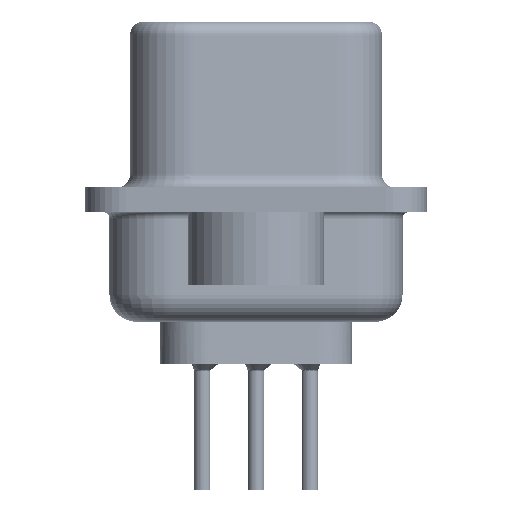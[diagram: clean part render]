
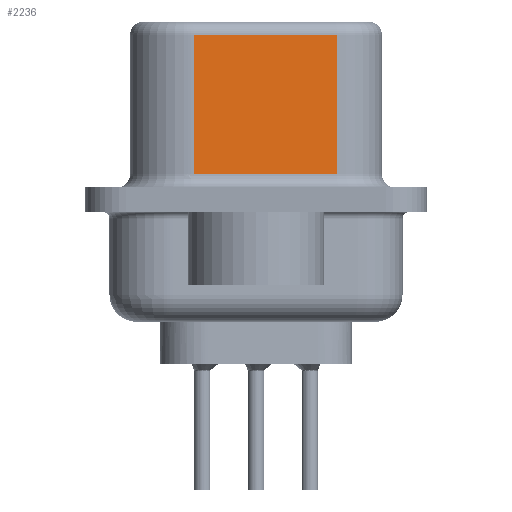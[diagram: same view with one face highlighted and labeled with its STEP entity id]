
A CAD part, left-side view. The second image highlights one B-rep face of the part: STEP entity #2236.
In plain terms, the highlighted planar face has unit normal (-0.985, -0.174, 0).
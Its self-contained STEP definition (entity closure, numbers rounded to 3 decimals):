
#2236 = ADVANCED_FACE ( 'NONE', ( #20825 ), #32775, .F. ) ;
#2850 = LINE ( 'NONE', #18222, #16570 ) ;
#3858 = ORIENTED_EDGE ( 'NONE', *, *, #23259, .T. ) ;
#4111 = EDGE_CURVE ( 'NONE', #20514, #13007, #37584, .T. ) ;
#10504 = CARTESIAN_POINT ( 'NONE',  ( 3.62, 2.293, 0.95 ) ) ;
#12948 = DIRECTION ( 'NONE',  ( 0., 0., -1. ) ) ;
#13007 = VERTEX_POINT ( 'NONE', #10504 ) ;
#13363 = CARTESIAN_POINT ( 'NONE',  ( 4.551, -2.987, 6.07 ) ) ;
#13517 = DIRECTION ( 'NONE',  ( 0., 0., -1. ) ) ;
#13564 = LINE ( 'NONE', #13363, #33303 ) ;
#15489 = VERTEX_POINT ( 'NONE', #37236 ) ;
#16129 = EDGE_CURVE ( 'NONE', #20421, #15489, #35183, .T. ) ;
#16496 = CARTESIAN_POINT ( 'NONE',  ( 4.551, -2.987, 6.57 ) ) ;
#16570 = VECTOR ( 'NONE', #27394, 1000. ) ;
#16953 = EDGE_LOOP ( 'NONE', ( #39284, #33028, #21821, #3858 ) ) ;
#18222 = CARTESIAN_POINT ( 'NONE',  ( 4.551, -2.987, 0.95 ) ) ;
#18298 = CARTESIAN_POINT ( 'NONE',  ( 4.551, -2.987, 6.07 ) ) ;
#20033 = EDGE_CURVE ( 'NONE', #20421, #20514, #13564, .T. ) ;
#20203 = CARTESIAN_POINT ( 'NONE',  ( 3.62, 2.293, 6.07 ) ) ;
#20421 = VERTEX_POINT ( 'NONE', #18298 ) ;
#20514 = VERTEX_POINT ( 'NONE', #20203 ) ;
#20825 = FACE_OUTER_BOUND ( 'NONE', #16953, .T. ) ;
#21821 = ORIENTED_EDGE ( 'NONE', *, *, #4111, .T. ) ;
#23259 = EDGE_CURVE ( 'NONE', #13007, #15489, #2850, .T. ) ;
#24296 = VECTOR ( 'NONE', #12948, 1000. ) ;
#24894 = CARTESIAN_POINT ( 'NONE',  ( 3.62, 2.293, 6.57 ) ) ;
#27004 = DIRECTION ( 'NONE',  ( -0.174, 0.985, 0. ) ) ;
#27394 = DIRECTION ( 'NONE',  ( 0.174, -0.985, 0. ) ) ;
#29694 = VECTOR ( 'NONE', #13517, 1000. ) ;
#31712 = AXIS2_PLACEMENT_3D ( 'NONE', #32964, #35159, #27004 ) ;
#32775 = PLANE ( 'NONE',  #31712 ) ;
#32964 = CARTESIAN_POINT ( 'NONE',  ( 4.551, -2.987, 6.57 ) ) ;
#33028 = ORIENTED_EDGE ( 'NONE', *, *, #20033, .T. ) ;
#33303 = VECTOR ( 'NONE', #35031, 1000. ) ;
#35031 = DIRECTION ( 'NONE',  ( -0.174, 0.985, 0. ) ) ;
#35159 = DIRECTION ( 'NONE',  ( 0.985, 0.174, 0. ) ) ;
#35183 = LINE ( 'NONE', #16496, #29694 ) ;
#37236 = CARTESIAN_POINT ( 'NONE',  ( 4.551, -2.987, 0.95 ) ) ;
#37584 = LINE ( 'NONE', #24894, #24296 ) ;
#39284 = ORIENTED_EDGE ( 'NONE', *, *, #16129, .F. ) ;
